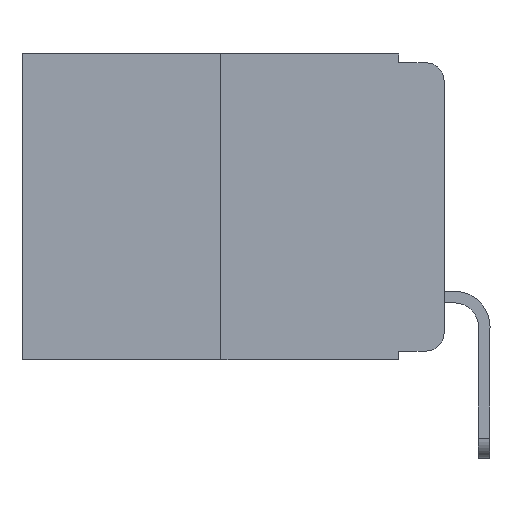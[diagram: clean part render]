
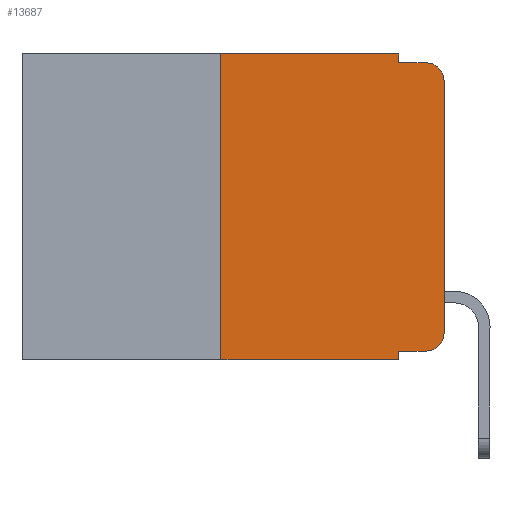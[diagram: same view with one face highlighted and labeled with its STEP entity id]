
A CAD part, left-side view. The second image highlights one B-rep face of the part: STEP entity #13687.
In plain terms, the highlighted planar face has unit normal (-1, 0, 0).
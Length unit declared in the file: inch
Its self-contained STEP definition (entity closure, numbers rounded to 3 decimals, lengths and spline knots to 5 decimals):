
#59 = VERTEX_POINT ( 'NONE', #4304 ) ;
#68 = ORIENTED_EDGE ( 'NONE', *, *, #7201, .F. ) ;
#74 = AXIS2_PLACEMENT_3D ( 'NONE', #10238, #311, #11775 ) ;
#311 = DIRECTION ( 'NONE',  ( -1., 0., 0. ) ) ;
#396 = ORIENTED_EDGE ( 'NONE', *, *, #13287, .F. ) ;
#422 = LINE ( 'NONE', #13006, #8798 ) ;
#606 = ORIENTED_EDGE ( 'NONE', *, *, #6376, .T. ) ;
#970 = DIRECTION ( 'NONE',  ( 1., 0., 0. ) ) ;
#1071 = EDGE_LOOP ( 'NONE', ( #5013, #606, #15783, #396, #3028, #68, #6225, #10263, #2516, #1072 ) ) ;
#1072 = ORIENTED_EDGE ( 'NONE', *, *, #10915, .T. ) ;
#1591 = CARTESIAN_POINT ( 'NONE',  ( 0., 0., -0.03 ) ) ;
#1933 = CARTESIAN_POINT ( 'NONE',  ( 0., 0.051, -0.343 ) ) ;
#2055 = VERTEX_POINT ( 'NONE', #20234 ) ;
#2298 = VERTEX_POINT ( 'NONE', #6366 ) ;
#2516 = ORIENTED_EDGE ( 'NONE', *, *, #11394, .T. ) ;
#2704 = LINE ( 'NONE', #15051, #10382 ) ;
#3028 = ORIENTED_EDGE ( 'NONE', *, *, #7602, .F. ) ;
#3069 = DIRECTION ( 'NONE',  ( 0., -1., 0. ) ) ;
#3442 = DIRECTION ( 'NONE',  ( 0., 0., 1. ) ) ;
#4304 = CARTESIAN_POINT ( 'NONE',  ( 0., 0.051, -0.333 ) ) ;
#4578 = VECTOR ( 'NONE', #13185, 39.37008 ) ;
#4636 = CARTESIAN_POINT ( 'NONE',  ( 0., 0.02, -0.313 ) ) ;
#5013 = ORIENTED_EDGE ( 'NONE', *, *, #18471, .T. ) ;
#5108 = LINE ( 'NONE', #5288, #4578 ) ;
#5288 = CARTESIAN_POINT ( 'NONE',  ( 0., 0.051, 0. ) ) ;
#5371 = LINE ( 'NONE', #9934, #8691 ) ;
#5665 = EDGE_CURVE ( 'NONE', #17721, #7281, #10718, .T. ) ;
#5723 = LINE ( 'NONE', #16742, #18055 ) ;
#5783 = VERTEX_POINT ( 'NONE', #1933 ) ;
#6225 = ORIENTED_EDGE ( 'NONE', *, *, #10553, .T. ) ;
#6326 = DIRECTION ( 'NONE',  ( 0., 0., -1. ) ) ;
#6366 = CARTESIAN_POINT ( 'NONE',  ( 0., 0.051, 0. ) ) ;
#6376 = EDGE_CURVE ( 'NONE', #11136, #7281, #6443, .T. ) ;
#6443 = CIRCLE ( 'NONE', #74, 0.02 ) ;
#6876 = DIRECTION ( 'NONE',  ( 0., -1., 0. ) ) ;
#6922 = EDGE_CURVE ( 'NONE', #59, #5783, #5108, .T. ) ;
#7201 = EDGE_CURVE ( 'NONE', #13501, #8999, #2704, .T. ) ;
#7281 = VERTEX_POINT ( 'NONE', #10771 ) ;
#7419 = CARTESIAN_POINT ( 'NONE',  ( 0., 0., -0.313 ) ) ;
#7602 = EDGE_CURVE ( 'NONE', #8999, #2298, #7684, .T. ) ;
#7684 = LINE ( 'NONE', #19097, #15824 ) ;
#8115 = CARTESIAN_POINT ( 'NONE',  ( 0., 0.051, -0.01 ) ) ;
#8617 = CARTESIAN_POINT ( 'NONE',  ( 0., 0.051, -0.01 ) ) ;
#8691 = VECTOR ( 'NONE', #11489, 39.37008 ) ;
#8798 = VECTOR ( 'NONE', #3442, 39.37008 ) ;
#8999 = VERTEX_POINT ( 'NONE', #9161 ) ;
#9161 = CARTESIAN_POINT ( 'NONE',  ( 0., 0.25, 0. ) ) ;
#9934 = CARTESIAN_POINT ( 'NONE',  ( 0., 0.051, 0. ) ) ;
#10238 = CARTESIAN_POINT ( 'NONE',  ( 0., 0.02, -0.03 ) ) ;
#10263 = ORIENTED_EDGE ( 'NONE', *, *, #6922, .F. ) ;
#10382 = VECTOR ( 'NONE', #10496, 39.37008 ) ;
#10496 = DIRECTION ( 'NONE',  ( 0., 0., 1. ) ) ;
#10553 = EDGE_CURVE ( 'NONE', #13501, #5783, #5723, .T. ) ;
#10718 = LINE ( 'NONE', #8115, #14242 ) ;
#10771 = CARTESIAN_POINT ( 'NONE',  ( 0., 0.02, -0.01 ) ) ;
#10915 = EDGE_CURVE ( 'NONE', #2055, #18092, #12398, .T. ) ;
#11136 = VERTEX_POINT ( 'NONE', #1591 ) ;
#11394 = EDGE_CURVE ( 'NONE', #59, #2055, #18725, .T. ) ;
#11489 = DIRECTION ( 'NONE',  ( 0., 0., -1. ) ) ;
#11775 = DIRECTION ( 'NONE',  ( 0., 0., -1. ) ) ;
#12398 = CIRCLE ( 'NONE', #17061, 0.02 ) ;
#13006 = CARTESIAN_POINT ( 'NONE',  ( 0., 0., 0. ) ) ;
#13185 = DIRECTION ( 'NONE',  ( 0., 0., -1. ) ) ;
#13287 = EDGE_CURVE ( 'NONE', #2298, #17721, #5371, .T. ) ;
#13368 = CARTESIAN_POINT ( 'NONE',  ( 0., 0.25, -0.343 ) ) ;
#13375 = DIRECTION ( 'NONE',  ( 0., -1., 0. ) ) ;
#13501 = VERTEX_POINT ( 'NONE', #13368 ) ;
#13655 = DIRECTION ( 'NONE',  ( 0., -1., 0. ) ) ;
#13687 = ADVANCED_FACE ( 'NONE', ( #15126 ), #15366, .F. ) ;
#13845 = CARTESIAN_POINT ( 'NONE',  ( 0., 0.473, 0. ) ) ;
#14242 = VECTOR ( 'NONE', #3069, 39.37008 ) ;
#15051 = CARTESIAN_POINT ( 'NONE',  ( 0., 0.25, 0. ) ) ;
#15126 = FACE_OUTER_BOUND ( 'NONE', #1071, .T. ) ;
#15366 = PLANE ( 'NONE',  #20014 ) ;
#15592 = DIRECTION ( 'NONE',  ( -1., 0., 0. ) ) ;
#15783 = ORIENTED_EDGE ( 'NONE', *, *, #5665, .F. ) ;
#15824 = VECTOR ( 'NONE', #6876, 39.37008 ) ;
#16386 = CARTESIAN_POINT ( 'NONE',  ( 0., 0.051, -0.333 ) ) ;
#16742 = CARTESIAN_POINT ( 'NONE',  ( 0., 0.473, -0.343 ) ) ;
#16925 = DIRECTION ( 'NONE',  ( 0., 0., -1. ) ) ;
#17061 = AXIS2_PLACEMENT_3D ( 'NONE', #4636, #15592, #6326 ) ;
#17721 = VERTEX_POINT ( 'NONE', #8617 ) ;
#18055 = VECTOR ( 'NONE', #13655, 39.37008 ) ;
#18092 = VERTEX_POINT ( 'NONE', #7419 ) ;
#18260 = VECTOR ( 'NONE', #13375, 39.37008 ) ;
#18471 = EDGE_CURVE ( 'NONE', #18092, #11136, #422, .T. ) ;
#18725 = LINE ( 'NONE', #16386, #18260 ) ;
#19097 = CARTESIAN_POINT ( 'NONE',  ( 0., 0.473, 0. ) ) ;
#20014 = AXIS2_PLACEMENT_3D ( 'NONE', #13845, #970, #16925 ) ;
#20234 = CARTESIAN_POINT ( 'NONE',  ( 0., 0.02, -0.333 ) ) ;
